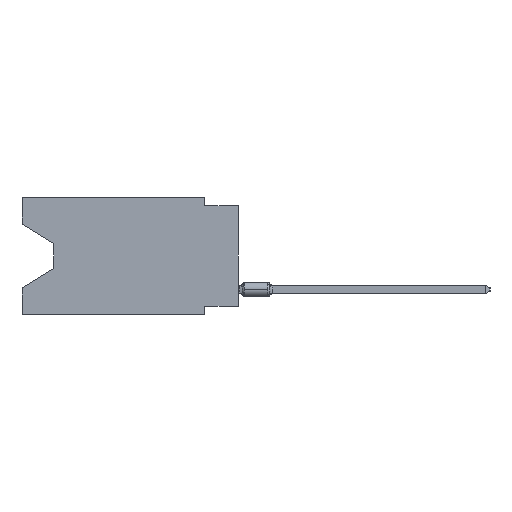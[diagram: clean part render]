
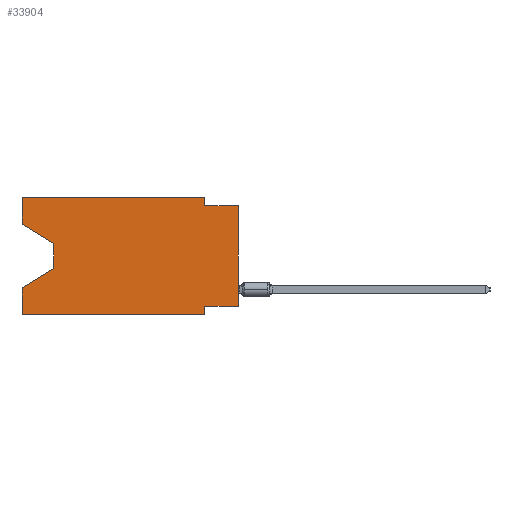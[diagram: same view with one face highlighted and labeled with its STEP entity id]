
A CAD part, left-side view. The second image highlights one B-rep face of the part: STEP entity #33904.
In plain terms, the highlighted planar face has unit normal (-1, 0, 0).
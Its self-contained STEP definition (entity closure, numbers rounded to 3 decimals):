
#570 = CARTESIAN_POINT ( 'NONE',  ( 0., 16.383, -2.038 ) ) ;
#1001 = EDGE_CURVE ( 'NONE', #3214, #37352, #22155, .T. ) ;
#1154 = VECTOR ( 'NONE', #59387, 1000. ) ;
#1187 = DIRECTION ( 'NONE',  ( 0., -0.855, -0.519 ) ) ;
#1472 = LINE ( 'NONE', #6805, #51411 ) ;
#3214 = VERTEX_POINT ( 'NONE', #57912 ) ;
#4272 = DIRECTION ( 'NONE',  ( 0., -1., 0. ) ) ;
#5898 = LINE ( 'NONE', #570, #57428 ) ;
#6805 = CARTESIAN_POINT ( 'NONE',  ( 0., 13.97, -3.505 ) ) ;
#6919 = VERTEX_POINT ( 'NONE', #23538 ) ;
#8073 = EDGE_CURVE ( 'NONE', #3214, #29190, #32448, .T. ) ;
#8520 = LINE ( 'NONE', #22274, #34889 ) ;
#9197 = CARTESIAN_POINT ( 'NONE',  ( 0., 16.383, -2.038 ) ) ;
#9358 = ORIENTED_EDGE ( 'NONE', *, *, #17541, .F. ) ;
#10557 = CARTESIAN_POINT ( 'NONE',  ( 0., 16.383, -8.89 ) ) ;
#10790 = VECTOR ( 'NONE', #4272, 1000. ) ;
#11011 = CARTESIAN_POINT ( 'NONE',  ( 0., 2.54, -0.635 ) ) ;
#13615 = VECTOR ( 'NONE', #38154, 1000. ) ;
#14004 = EDGE_CURVE ( 'NONE', #29190, #25608, #20534, .T. ) ;
#14619 = CARTESIAN_POINT ( 'NONE',  ( 0., 0., -8.255 ) ) ;
#15657 = ORIENTED_EDGE ( 'NONE', *, *, #16114, .T. ) ;
#15770 = VERTEX_POINT ( 'NONE', #18934 ) ;
#16114 = EDGE_CURVE ( 'NONE', #31116, #6919, #33594, .T. ) ;
#17541 = EDGE_CURVE ( 'NONE', #47457, #27334, #57222, .T. ) ;
#17874 = EDGE_CURVE ( 'NONE', #18990, #25608, #49724, .T. ) ;
#18749 = FACE_OUTER_BOUND ( 'NONE', #29104, .T. ) ;
#18934 = CARTESIAN_POINT ( 'NONE',  ( 0., 16.383, 0. ) ) ;
#18990 = VERTEX_POINT ( 'NONE', #10557 ) ;
#19254 = VECTOR ( 'NONE', #55527, 1000. ) ;
#20534 = LINE ( 'NONE', #58681, #19254 ) ;
#20670 = ORIENTED_EDGE ( 'NONE', *, *, #60130, .F. ) ;
#20991 = EDGE_CURVE ( 'NONE', #27334, #37352, #24735, .T. ) ;
#21907 = ORIENTED_EDGE ( 'NONE', *, *, #30854, .T. ) ;
#22148 = EDGE_CURVE ( 'NONE', #18990, #6919, #8520, .T. ) ;
#22155 = LINE ( 'NONE', #40302, #1154 ) ;
#22274 = CARTESIAN_POINT ( 'NONE',  ( 0., 16.383, 0. ) ) ;
#22789 = VECTOR ( 'NONE', #47540, 1000. ) ;
#23538 = CARTESIAN_POINT ( 'NONE',  ( 0., 16.383, -6.852 ) ) ;
#23608 = CARTESIAN_POINT ( 'NONE',  ( 0., 16.383, 0. ) ) ;
#24415 = CARTESIAN_POINT ( 'NONE',  ( 0., 0., -0.635 ) ) ;
#24735 = LINE ( 'NONE', #24415, #22789 ) ;
#25608 = VERTEX_POINT ( 'NONE', #60675 ) ;
#26733 = AXIS2_PLACEMENT_3D ( 'NONE', #36888, #32201, #26904 ) ;
#26857 = CARTESIAN_POINT ( 'NONE',  ( 0., 2.54, -8.255 ) ) ;
#26904 = DIRECTION ( 'NONE',  ( 0., 0., -1. ) ) ;
#27334 = VERTEX_POINT ( 'NONE', #11011 ) ;
#27566 = VECTOR ( 'NONE', #47114, 1000. ) ;
#28052 = ORIENTED_EDGE ( 'NONE', *, *, #14004, .F. ) ;
#29104 = EDGE_LOOP ( 'NONE', ( #61154, #21907, #15657, #53822, #35681, #28052, #37101, #31514, #36588, #9358, #20670, #40015 ) ) ;
#29190 = VERTEX_POINT ( 'NONE', #26857 ) ;
#29206 = DIRECTION ( 'NONE',  ( 0., 0.855, -0.519 ) ) ;
#30651 = CARTESIAN_POINT ( 'NONE',  ( 0., 16.383, -8.89 ) ) ;
#30854 = EDGE_CURVE ( 'NONE', #30923, #31116, #1472, .T. ) ;
#30923 = VERTEX_POINT ( 'NONE', #44597 ) ;
#31116 = VERTEX_POINT ( 'NONE', #37058 ) ;
#31514 = ORIENTED_EDGE ( 'NONE', *, *, #1001, .T. ) ;
#32201 = DIRECTION ( 'NONE',  ( 1., 0., 0. ) ) ;
#32448 = LINE ( 'NONE', #14619, #27566 ) ;
#33594 = LINE ( 'NONE', #52986, #60397 ) ;
#33904 = ADVANCED_FACE ( 'NONE', ( #18749 ), #47169, .F. ) ;
#33923 = CARTESIAN_POINT ( 'NONE',  ( 0., 0., -0.635 ) ) ;
#34889 = VECTOR ( 'NONE', #55421, 1000. ) ;
#35681 = ORIENTED_EDGE ( 'NONE', *, *, #17874, .T. ) ;
#36013 = EDGE_CURVE ( 'NONE', #55636, #15770, #38271, .T. ) ;
#36588 = ORIENTED_EDGE ( 'NONE', *, *, #20991, .F. ) ;
#36888 = CARTESIAN_POINT ( 'NONE',  ( 0., 16.383, 0. ) ) ;
#37058 = CARTESIAN_POINT ( 'NONE',  ( 0., 13.97, -5.385 ) ) ;
#37101 = ORIENTED_EDGE ( 'NONE', *, *, #8073, .F. ) ;
#37292 = VECTOR ( 'NONE', #43259, 1000. ) ;
#37352 = VERTEX_POINT ( 'NONE', #33923 ) ;
#38154 = DIRECTION ( 'NONE',  ( 0., 0., -1. ) ) ;
#38271 = LINE ( 'NONE', #23608, #37292 ) ;
#40015 = ORIENTED_EDGE ( 'NONE', *, *, #36013, .F. ) ;
#40302 = CARTESIAN_POINT ( 'NONE',  ( 0., 0., 0. ) ) ;
#40636 = VECTOR ( 'NONE', #54411, 1000. ) ;
#43259 = DIRECTION ( 'NONE',  ( 0., 0., 1. ) ) ;
#44304 = CARTESIAN_POINT ( 'NONE',  ( 0., 2.54, 0. ) ) ;
#44597 = CARTESIAN_POINT ( 'NONE',  ( 0., 13.97, -3.505 ) ) ;
#47084 = CARTESIAN_POINT ( 'NONE',  ( 0., 16.383, 0. ) ) ;
#47114 = DIRECTION ( 'NONE',  ( 0., 1., 0. ) ) ;
#47169 = PLANE ( 'NONE',  #26733 ) ;
#47412 = EDGE_CURVE ( 'NONE', #55636, #30923, #5898, .T. ) ;
#47457 = VERTEX_POINT ( 'NONE', #44304 ) ;
#47540 = DIRECTION ( 'NONE',  ( 0., -1., 0. ) ) ;
#49724 = LINE ( 'NONE', #30651, #40636 ) ;
#51411 = VECTOR ( 'NONE', #58055, 1000. ) ;
#52986 = CARTESIAN_POINT ( 'NONE',  ( 0., 13.97, -5.385 ) ) ;
#53822 = ORIENTED_EDGE ( 'NONE', *, *, #22148, .F. ) ;
#54411 = DIRECTION ( 'NONE',  ( 0., -1., 0. ) ) ;
#55421 = DIRECTION ( 'NONE',  ( 0., 0., 1. ) ) ;
#55527 = DIRECTION ( 'NONE',  ( 0., 0., -1. ) ) ;
#55636 = VERTEX_POINT ( 'NONE', #9197 ) ;
#56634 = CARTESIAN_POINT ( 'NONE',  ( 0., 2.54, 0. ) ) ;
#57222 = LINE ( 'NONE', #56634, #13615 ) ;
#57428 = VECTOR ( 'NONE', #1187, 1000. ) ;
#57912 = CARTESIAN_POINT ( 'NONE',  ( 0., 0., -8.255 ) ) ;
#58055 = DIRECTION ( 'NONE',  ( 0., 0., -1. ) ) ;
#58681 = CARTESIAN_POINT ( 'NONE',  ( 0., 2.54, -8.89 ) ) ;
#59387 = DIRECTION ( 'NONE',  ( 0., 0., 1. ) ) ;
#60130 = EDGE_CURVE ( 'NONE', #15770, #47457, #61152, .T. ) ;
#60397 = VECTOR ( 'NONE', #29206, 1000. ) ;
#60675 = CARTESIAN_POINT ( 'NONE',  ( 0., 2.54, -8.89 ) ) ;
#61152 = LINE ( 'NONE', #47084, #10790 ) ;
#61154 = ORIENTED_EDGE ( 'NONE', *, *, #47412, .T. ) ;
